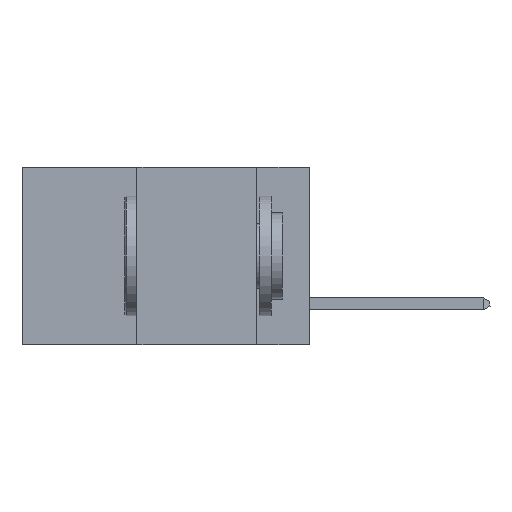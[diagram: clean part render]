
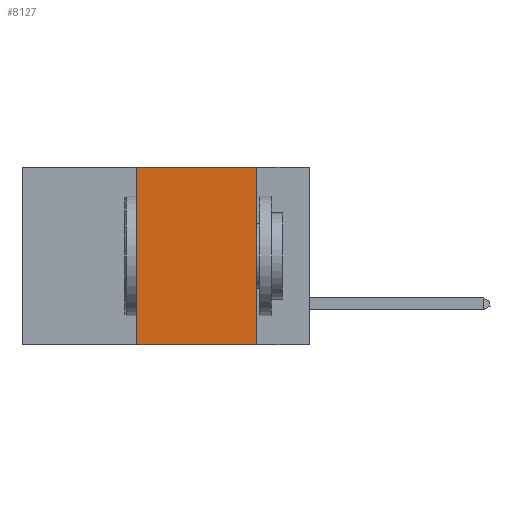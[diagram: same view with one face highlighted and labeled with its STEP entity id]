
A CAD part, left-side view. The second image highlights one B-rep face of the part: STEP entity #8127.
In plain terms, the highlighted planar face has unit normal (-1, 0, 0).
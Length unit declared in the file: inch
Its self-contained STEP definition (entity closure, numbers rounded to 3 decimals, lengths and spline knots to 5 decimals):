
#120 = CARTESIAN_POINT ( 'NONE',  ( 0., 0.36, 0. ) ) ;
#1315 = FACE_OUTER_BOUND ( 'NONE', #11742, .T. ) ;
#1562 = DIRECTION ( 'NONE',  ( 0., 0., 1. ) ) ;
#1757 = LINE ( 'NONE', #7086, #8537 ) ;
#2154 = PLANE ( 'NONE',  #4306 ) ;
#2349 = CARTESIAN_POINT ( 'NONE',  ( 0., 0.6, 0. ) ) ;
#2416 = CARTESIAN_POINT ( 'NONE',  ( 0., 0.11, 0. ) ) ;
#2713 = VECTOR ( 'NONE', #6860, 39.37008 ) ;
#2786 = ORIENTED_EDGE ( 'NONE', *, *, #6789, .T. ) ;
#3049 = EDGE_CURVE ( 'NONE', #8467, #4247, #9760, .T. ) ;
#3158 = DIRECTION ( 'NONE',  ( 1., 0., 0. ) ) ;
#3949 = DIRECTION ( 'NONE',  ( 0., 0., -1. ) ) ;
#4090 = ORIENTED_EDGE ( 'NONE', *, *, #9113, .F. ) ;
#4247 = VERTEX_POINT ( 'NONE', #2416 ) ;
#4306 = AXIS2_PLACEMENT_3D ( 'NONE', #8608, #3158, #9543 ) ;
#4648 = CARTESIAN_POINT ( 'NONE',  ( 0., 0.11, -0.37 ) ) ;
#5014 = VECTOR ( 'NONE', #7368, 39.37008 ) ;
#6137 = ORIENTED_EDGE ( 'NONE', *, *, #8711, .F. ) ;
#6184 = CARTESIAN_POINT ( 'NONE',  ( 0., 0.36, -0.37 ) ) ;
#6789 = EDGE_CURVE ( 'NONE', #9707, #9333, #9912, .T. ) ;
#6860 = DIRECTION ( 'NONE',  ( 0., -1., 0. ) ) ;
#7086 = CARTESIAN_POINT ( 'NONE',  ( 0., 0.36, 0. ) ) ;
#7368 = DIRECTION ( 'NONE',  ( 0., -1., 0. ) ) ;
#7537 = VECTOR ( 'NONE', #3949, 39.37008 ) ;
#7634 = ORIENTED_EDGE ( 'NONE', *, *, #3049, .F. ) ;
#8127 = ADVANCED_FACE ( 'NONE', ( #1315 ), #2154, .F. ) ;
#8467 = VERTEX_POINT ( 'NONE', #120 ) ;
#8537 = VECTOR ( 'NONE', #1562, 39.37008 ) ;
#8608 = CARTESIAN_POINT ( 'NONE',  ( 0., 0.6, 0. ) ) ;
#8711 = EDGE_CURVE ( 'NONE', #9707, #8467, #1757, .T. ) ;
#9110 = CARTESIAN_POINT ( 'NONE',  ( 0., 0.6, -0.37 ) ) ;
#9113 = EDGE_CURVE ( 'NONE', #4247, #9333, #9837, .T. ) ;
#9333 = VERTEX_POINT ( 'NONE', #4648 ) ;
#9543 = DIRECTION ( 'NONE',  ( 0., 0., -1. ) ) ;
#9544 = CARTESIAN_POINT ( 'NONE',  ( 0., 0.11, 0. ) ) ;
#9707 = VERTEX_POINT ( 'NONE', #6184 ) ;
#9760 = LINE ( 'NONE', #2349, #2713 ) ;
#9837 = LINE ( 'NONE', #9544, #7537 ) ;
#9912 = LINE ( 'NONE', #9110, #5014 ) ;
#11742 = EDGE_LOOP ( 'NONE', ( #4090, #7634, #6137, #2786 ) ) ;
